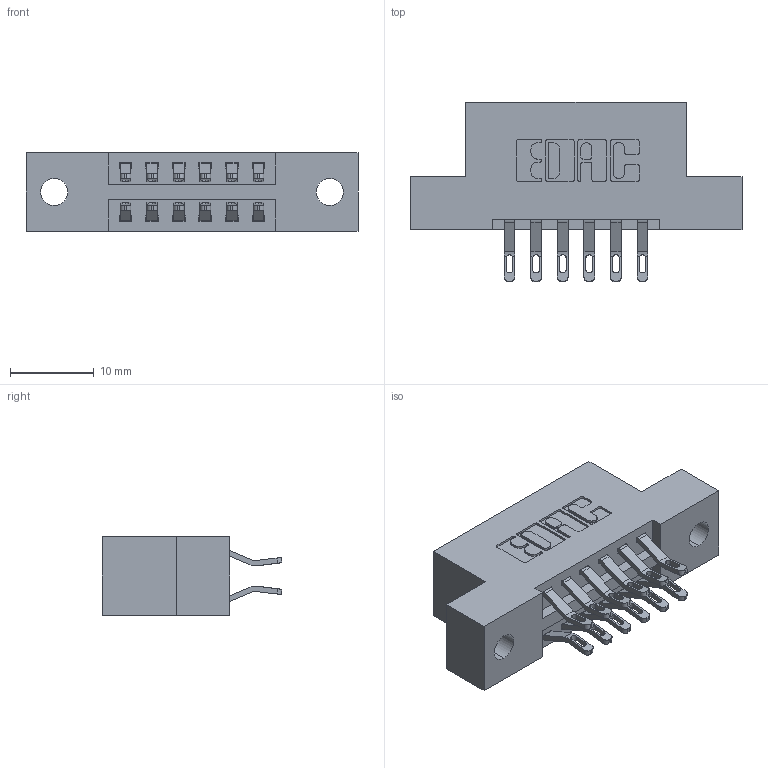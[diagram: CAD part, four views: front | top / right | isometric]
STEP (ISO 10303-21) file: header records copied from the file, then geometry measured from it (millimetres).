
FILE_DESCRIPTION (( 'STEP AP203' ), '1' );
FILE_NAME ('396-012-555-202.STEP', '2019-10-29T19:35:25', ( '' ), ( '' ), 'SwSTEP 2.0', 'SolidWorks 2016', '' );
FILE_SCHEMA (( 'CONFIG_CONTROL_DESIGN' ));
Length unit declared in the file: inch
Products named in the file (3): 396-012-555-202; 345-292-001_555 Tail; 346 Part_Flush Mounting Lugs - 0.128 Dia
Assembly tree (13 placements, depth 2):
  396-012-555-202
    346 Part_Flush Mounting Lugs - 0.128 Dia
    345-292-001_555 Tail  x12
Bounding box: 39.62 x 21.46 x 9.4 mm (x, y, z)
Volume: 3582.4 mm3; surface area: 4213.2 mm2
Topology: 13 solids, 13 shells, 818 faces, 2525 edges, 1682 vertices
Faces by surface type: plane 472, cylinder 346
Entity records: 9091 total; most frequent: CARTESIAN_POINT 1582, ORIENTED_EDGE 1486, DIRECTION 1415, EDGE_CURVE 743, LINE 567, VECTOR 567, VERTEX_POINT 494, AXIS2_PLACEMENT_3D 424
